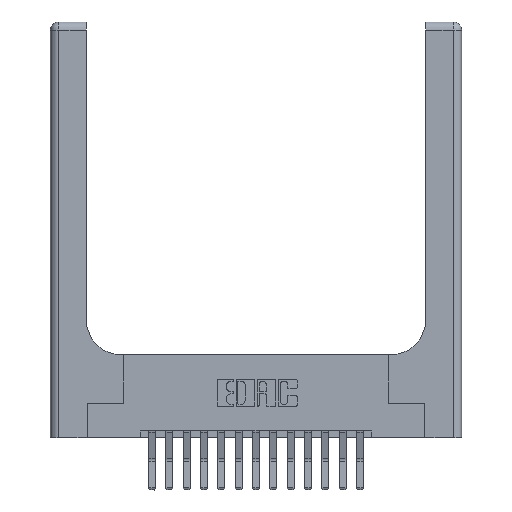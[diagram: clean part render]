
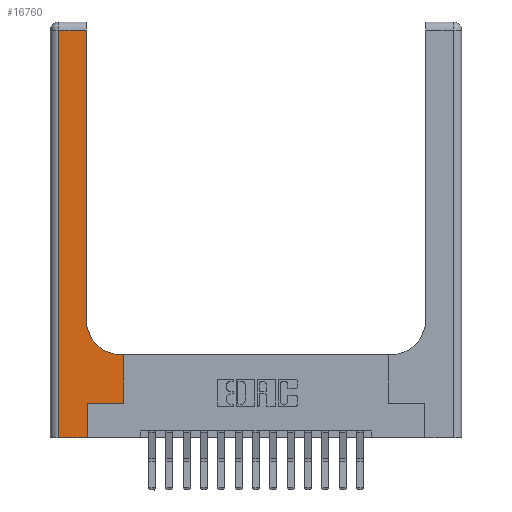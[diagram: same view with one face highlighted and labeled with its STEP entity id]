
A CAD part, top view. The second image highlights one B-rep face of the part: STEP entity #16760.
In plain terms, the highlighted planar face has unit normal (0, 0, 1).
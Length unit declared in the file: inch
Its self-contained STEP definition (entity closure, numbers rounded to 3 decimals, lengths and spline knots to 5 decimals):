
#135 = VERTEX_POINT ( 'NONE', #14569 ) ;
#1212 = LINE ( 'NONE', #9680, #16378 ) ;
#1377 = DIRECTION ( 'NONE',  ( -1., 0., 0. ) ) ;
#1712 = VERTEX_POINT ( 'NONE', #16417 ) ;
#1829 = DIRECTION ( 'NONE',  ( -1., 0., 0. ) ) ;
#1895 = EDGE_CURVE ( 'NONE', #4895, #2597, #4174, .T. ) ;
#2145 = EDGE_CURVE ( 'NONE', #6731, #13987, #1212, .T. ) ;
#2229 = EDGE_CURVE ( 'NONE', #10535, #6731, #15503, .T. ) ;
#2542 = VERTEX_POINT ( 'NONE', #10365 ) ;
#2597 = VERTEX_POINT ( 'NONE', #5290 ) ;
#3375 = LINE ( 'NONE', #5465, #3590 ) ;
#3378 = CARTESIAN_POINT ( 'NONE',  ( 0.06, 0., 0.37 ) ) ;
#3513 = CARTESIAN_POINT ( 'NONE',  ( 0.06, 2.94, 0.37 ) ) ;
#3590 = VECTOR ( 'NONE', #1377, 39.37008 ) ;
#4174 = LINE ( 'NONE', #11608, #5908 ) ;
#4539 = ORIENTED_EDGE ( 'NONE', *, *, #1895, .T. ) ;
#4620 = EDGE_CURVE ( 'NONE', #2542, #1712, #17567, .T. ) ;
#4823 = ORIENTED_EDGE ( 'NONE', *, *, #8057, .T. ) ;
#4895 = VERTEX_POINT ( 'NONE', #10283 ) ;
#5290 = CARTESIAN_POINT ( 'NONE',  ( 0.528, 0.6, 0.37 ) ) ;
#5465 = CARTESIAN_POINT ( 'NONE',  ( 0., 2.94, 0.37 ) ) ;
#5879 = CARTESIAN_POINT ( 'NONE',  ( 0., 3., 0.37 ) ) ;
#5908 = VECTOR ( 'NONE', #13042, 39.37008 ) ;
#5942 = EDGE_LOOP ( 'NONE', ( #15265, #4823, #9854, #12573, #9048, #7417, #4539, #13460, #14909 ) ) ;
#6109 = CARTESIAN_POINT ( 'NONE',  ( 0.06, 3., 0.37 ) ) ;
#6731 = VERTEX_POINT ( 'NONE', #3378 ) ;
#6883 = EDGE_CURVE ( 'NONE', #2597, #135, #14755, .T. ) ;
#6894 = VECTOR ( 'NONE', #17658, 39.37008 ) ;
#7031 = EDGE_CURVE ( 'NONE', #13987, #7687, #12836, .T. ) ;
#7137 = CARTESIAN_POINT ( 'NONE',  ( 0.265, 0., 0.37 ) ) ;
#7344 = DIRECTION ( 'NONE',  ( 0., 0., -1. ) ) ;
#7417 = ORIENTED_EDGE ( 'NONE', *, *, #13953, .T. ) ;
#7419 = CARTESIAN_POINT ( 'NONE',  ( 0.265, 0.25, 0.37 ) ) ;
#7687 = VERTEX_POINT ( 'NONE', #7419 ) ;
#8057 = EDGE_CURVE ( 'NONE', #1712, #10535, #3375, .T. ) ;
#8236 = CARTESIAN_POINT ( 'NONE',  ( 0.265, 0., 0.37 ) ) ;
#8765 = DIRECTION ( 'NONE',  ( 1., 0., 0. ) ) ;
#9048 = ORIENTED_EDGE ( 'NONE', *, *, #7031, .T. ) ;
#9105 = AXIS2_PLACEMENT_3D ( 'NONE', #11296, #7344, #12851 ) ;
#9574 = CARTESIAN_POINT ( 'NONE',  ( 0.26, 3., 0.37 ) ) ;
#9680 = CARTESIAN_POINT ( 'NONE',  ( 0., 0., 0.37 ) ) ;
#9854 = ORIENTED_EDGE ( 'NONE', *, *, #2229, .T. ) ;
#10101 = DIRECTION ( 'NONE',  ( 0., 0., -1. ) ) ;
#10283 = CARTESIAN_POINT ( 'NONE',  ( 0.528, 0.25, 0.37 ) ) ;
#10365 = CARTESIAN_POINT ( 'NONE',  ( 0.26, 0.85, 0.37 ) ) ;
#10535 = VERTEX_POINT ( 'NONE', #3513 ) ;
#10843 = VECTOR ( 'NONE', #14070, 39.37008 ) ;
#11296 = CARTESIAN_POINT ( 'NONE',  ( 0.51, 0.85, 0.37 ) ) ;
#11608 = CARTESIAN_POINT ( 'NONE',  ( 0.528, 0.25, 0.37 ) ) ;
#11786 = VECTOR ( 'NONE', #14928, 39.37008 ) ;
#12327 = DIRECTION ( 'NONE',  ( -1., 0., 0. ) ) ;
#12377 = EDGE_CURVE ( 'NONE', #135, #2542, #16330, .T. ) ;
#12573 = ORIENTED_EDGE ( 'NONE', *, *, #2145, .T. ) ;
#12637 = LINE ( 'NONE', #17592, #11786 ) ;
#12836 = LINE ( 'NONE', #7137, #15371 ) ;
#12851 = DIRECTION ( 'NONE',  ( 1., 0., 0. ) ) ;
#13042 = DIRECTION ( 'NONE',  ( 0., 1., 0. ) ) ;
#13047 = VECTOR ( 'NONE', #12327, 39.37008 ) ;
#13460 = ORIENTED_EDGE ( 'NONE', *, *, #6883, .T. ) ;
#13953 = EDGE_CURVE ( 'NONE', #7687, #4895, #12637, .T. ) ;
#13987 = VERTEX_POINT ( 'NONE', #8236 ) ;
#14070 = DIRECTION ( 'NONE',  ( 0., -1., 0. ) ) ;
#14569 = CARTESIAN_POINT ( 'NONE',  ( 0.51, 0.6, 0.37 ) ) ;
#14755 = LINE ( 'NONE', #15006, #13047 ) ;
#14909 = ORIENTED_EDGE ( 'NONE', *, *, #12377, .T. ) ;
#14928 = DIRECTION ( 'NONE',  ( 1., 0., 0. ) ) ;
#15006 = CARTESIAN_POINT ( 'NONE',  ( 0.26, 0.6, 0.37 ) ) ;
#15265 = ORIENTED_EDGE ( 'NONE', *, *, #4620, .T. ) ;
#15371 = VECTOR ( 'NONE', #16692, 39.37008 ) ;
#15503 = LINE ( 'NONE', #6109, #10843 ) ;
#15555 = PLANE ( 'NONE',  #17137 ) ;
#16330 = CIRCLE ( 'NONE', #9105, 0.25 ) ;
#16378 = VECTOR ( 'NONE', #8765, 39.37008 ) ;
#16417 = CARTESIAN_POINT ( 'NONE',  ( 0.26, 2.94, 0.37 ) ) ;
#16692 = DIRECTION ( 'NONE',  ( 0., 1., 0. ) ) ;
#16760 = ADVANCED_FACE ( 'NONE', ( #16925 ), #15555, .F. ) ;
#16925 = FACE_OUTER_BOUND ( 'NONE', #5942, .T. ) ;
#17137 = AXIS2_PLACEMENT_3D ( 'NONE', #5879, #10101, #1829 ) ;
#17567 = LINE ( 'NONE', #9574, #6894 ) ;
#17592 = CARTESIAN_POINT ( 'NONE',  ( 0.265, 0.25, 0.37 ) ) ;
#17658 = DIRECTION ( 'NONE',  ( 0., 1., 0. ) ) ;
